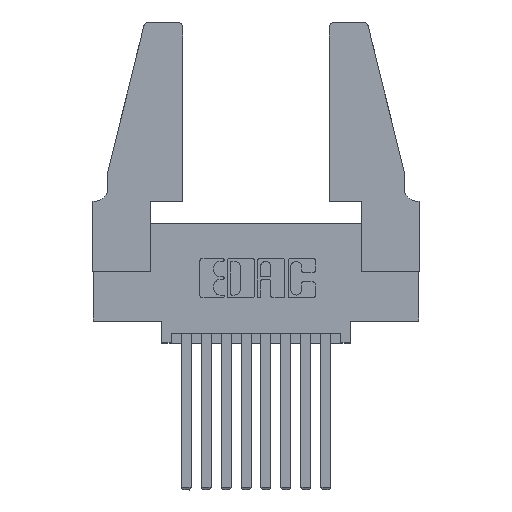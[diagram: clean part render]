
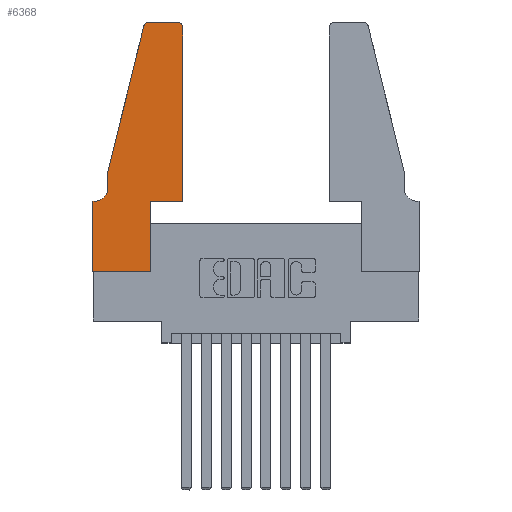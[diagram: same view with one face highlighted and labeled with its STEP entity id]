
A CAD part, top view. The second image highlights one B-rep face of the part: STEP entity #6368.
In plain terms, the highlighted planar face has unit normal (0, 0, 1).
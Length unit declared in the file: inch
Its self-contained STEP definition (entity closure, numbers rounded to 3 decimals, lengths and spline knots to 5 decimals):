
#100 = ORIENTED_EDGE ( 'NONE', *, *, #12266, .T. ) ;
#156 = VECTOR ( 'NONE', #745, 39.37008 ) ;
#252 = VERTEX_POINT ( 'NONE', #7907 ) ;
#286 = DIRECTION ( 'NONE',  ( -0.239, -0.971, 0. ) ) ;
#383 = CARTESIAN_POINT ( 'NONE',  ( 0., 0., 0.37 ) ) ;
#745 = DIRECTION ( 'NONE',  ( -1., 0., 0. ) ) ;
#772 = CARTESIAN_POINT ( 'NONE',  ( 0.0755, 0.5, 0.37 ) ) ;
#869 = CARTESIAN_POINT ( 'NONE',  ( 0.4205, 1.22, 0.37 ) ) ;
#890 = AXIS2_PLACEMENT_3D ( 'NONE', #2782, #3839, #6799 ) ;
#1001 = CARTESIAN_POINT ( 'NONE',  ( 0.284, 1.25, 0.37 ) ) ;
#1267 = CARTESIAN_POINT ( 'NONE',  ( 0.4505, 1.22, 0.37 ) ) ;
#1347 = ORIENTED_EDGE ( 'NONE', *, *, #10924, .T. ) ;
#1435 = VECTOR ( 'NONE', #3525, 39.37008 ) ;
#1840 = CARTESIAN_POINT ( 'NONE',  ( 0.4505, 0.35, 0.37 ) ) ;
#1850 = LINE ( 'NONE', #772, #5919 ) ;
#1855 = EDGE_CURVE ( 'NONE', #7371, #9687, #1850, .T. ) ;
#1903 = CARTESIAN_POINT ( 'NONE',  ( 0.0755, 0.5, 0.37 ) ) ;
#2557 = CARTESIAN_POINT ( 'NONE',  ( 0.2865, 0.35, 0.37 ) ) ;
#2782 = CARTESIAN_POINT ( 'NONE',  ( 0.0055, 0.42, 0.37 ) ) ;
#2971 = LINE ( 'NONE', #7767, #8925 ) ;
#3011 = CIRCLE ( 'NONE', #890, 0.07 ) ;
#3025 = CIRCLE ( 'NONE', #7605, 0.03 ) ;
#3317 = EDGE_CURVE ( 'NONE', #11089, #12493, #10253, .T. ) ;
#3330 = CARTESIAN_POINT ( 'NONE',  ( 0.284, 1.22, 0.37 ) ) ;
#3419 = DIRECTION ( 'NONE',  ( 1., 0., 0. ) ) ;
#3525 = DIRECTION ( 'NONE',  ( 0., -1., 0. ) ) ;
#3647 = CARTESIAN_POINT ( 'NONE',  ( 0., 0.35, 0.37 ) ) ;
#3662 = VECTOR ( 'NONE', #10313, 39.37008 ) ;
#3750 = VECTOR ( 'NONE', #286, 39.37008 ) ;
#3831 = PLANE ( 'NONE',  #8722 ) ;
#3839 = DIRECTION ( 'NONE',  ( 0., 0., -1. ) ) ;
#3955 = AXIS2_PLACEMENT_3D ( 'NONE', #3330, #9452, #3419 ) ;
#4276 = CARTESIAN_POINT ( 'NONE',  ( 0., 0.35, 0.37 ) ) ;
#4323 = VECTOR ( 'NONE', #5979, 39.37008 ) ;
#4641 = ORIENTED_EDGE ( 'NONE', *, *, #11639, .T. ) ;
#5005 = CARTESIAN_POINT ( 'NONE',  ( 0.0055, 0.35, 0.37 ) ) ;
#5473 = LINE ( 'NONE', #6293, #3750 ) ;
#5795 = DIRECTION ( 'NONE',  ( 0., 0., 1. ) ) ;
#5812 = DIRECTION ( 'NONE',  ( 1., 0., 0. ) ) ;
#5919 = VECTOR ( 'NONE', #11779, 39.37008 ) ;
#5979 = DIRECTION ( 'NONE',  ( -1., 0., 0. ) ) ;
#6196 = VECTOR ( 'NONE', #12557, 39.37008 ) ;
#6293 = CARTESIAN_POINT ( 'NONE',  ( 0.0755, 0.5, 0.37 ) ) ;
#6336 = CARTESIAN_POINT ( 'NONE',  ( 0.4505, 0.35, 0.37 ) ) ;
#6368 = ADVANCED_FACE ( 'NONE', ( #8621 ), #3831, .T. ) ;
#6444 = LINE ( 'NONE', #9816, #156 ) ;
#6614 = EDGE_CURVE ( 'NONE', #12202, #7371, #5473, .T. ) ;
#6792 = ORIENTED_EDGE ( 'NONE', *, *, #7419, .T. ) ;
#6795 = CARTESIAN_POINT ( 'NONE',  ( 0.2605, 1.25, 0.37 ) ) ;
#6799 = DIRECTION ( 'NONE',  ( -1., 0., 0. ) ) ;
#7087 = ORIENTED_EDGE ( 'NONE', *, *, #3317, .T. ) ;
#7198 = ORIENTED_EDGE ( 'NONE', *, *, #8998, .T. ) ;
#7279 = EDGE_CURVE ( 'NONE', #8082, #12202, #12154, .T. ) ;
#7371 = VERTEX_POINT ( 'NONE', #1903 ) ;
#7419 = EDGE_CURVE ( 'NONE', #9749, #12370, #2971, .T. ) ;
#7465 = ORIENTED_EDGE ( 'NONE', *, *, #1855, .T. ) ;
#7605 = AXIS2_PLACEMENT_3D ( 'NONE', #869, #12843, #5812 ) ;
#7742 = CARTESIAN_POINT ( 'NONE',  ( 0.25487, 1.22718, 0.37 ) ) ;
#7767 = CARTESIAN_POINT ( 'NONE',  ( 0., 0., 0.37 ) ) ;
#7865 = ORIENTED_EDGE ( 'NONE', *, *, #10103, .T. ) ;
#7907 = CARTESIAN_POINT ( 'NONE',  ( 0.4205, 1.25, 0.37 ) ) ;
#8082 = VERTEX_POINT ( 'NONE', #1001 ) ;
#8331 = ORIENTED_EDGE ( 'NONE', *, *, #12704, .T. ) ;
#8621 = FACE_OUTER_BOUND ( 'NONE', #10375, .T. ) ;
#8636 = CARTESIAN_POINT ( 'NONE',  ( 0.4505, 0.35, 0.37 ) ) ;
#8722 = AXIS2_PLACEMENT_3D ( 'NONE', #3647, #5795, #9675 ) ;
#8925 = VECTOR ( 'NONE', #9840, 39.37008 ) ;
#8992 = LINE ( 'NONE', #6336, #3662 ) ;
#8998 = EDGE_CURVE ( 'NONE', #12370, #10031, #10120, .T. ) ;
#9105 = CARTESIAN_POINT ( 'NONE',  ( 0.0755, 0.42, 0.37 ) ) ;
#9452 = DIRECTION ( 'NONE',  ( 0., 0., 1. ) ) ;
#9516 = CARTESIAN_POINT ( 'NONE',  ( 0., 0., 0.37 ) ) ;
#9537 = DIRECTION ( 'NONE',  ( 0., 1., 0. ) ) ;
#9675 = DIRECTION ( 'NONE',  ( 1., 0., 0. ) ) ;
#9687 = VERTEX_POINT ( 'NONE', #9105 ) ;
#9749 = VERTEX_POINT ( 'NONE', #383 ) ;
#9816 = CARTESIAN_POINT ( 'NONE',  ( 0.0755, 0.35, 0.37 ) ) ;
#9840 = DIRECTION ( 'NONE',  ( 1., 0., 0. ) ) ;
#10031 = VERTEX_POINT ( 'NONE', #10703 ) ;
#10103 = EDGE_CURVE ( 'NONE', #252, #8082, #10875, .T. ) ;
#10120 = LINE ( 'NONE', #2557, #11533 ) ;
#10202 = ORIENTED_EDGE ( 'NONE', *, *, #11139, .T. ) ;
#10253 = LINE ( 'NONE', #8636, #6196 ) ;
#10313 = DIRECTION ( 'NONE',  ( 1., 0., 0. ) ) ;
#10375 = EDGE_LOOP ( 'NONE', ( #7865, #11960, #12060, #7465, #4641, #100, #8331, #6792, #7198, #1347, #7087, #10202 ) ) ;
#10703 = CARTESIAN_POINT ( 'NONE',  ( 0.2865, 0.35, 0.37 ) ) ;
#10709 = VERTEX_POINT ( 'NONE', #5005 ) ;
#10875 = LINE ( 'NONE', #6795, #4323 ) ;
#10924 = EDGE_CURVE ( 'NONE', #10031, #11089, #8992, .T. ) ;
#11089 = VERTEX_POINT ( 'NONE', #1840 ) ;
#11139 = EDGE_CURVE ( 'NONE', #12493, #252, #3025, .T. ) ;
#11533 = VECTOR ( 'NONE', #9537, 39.37008 ) ;
#11639 = EDGE_CURVE ( 'NONE', #9687, #10709, #3011, .T. ) ;
#11779 = DIRECTION ( 'NONE',  ( 0., -1., 0. ) ) ;
#11897 = VERTEX_POINT ( 'NONE', #4276 ) ;
#11960 = ORIENTED_EDGE ( 'NONE', *, *, #7279, .T. ) ;
#12055 = CARTESIAN_POINT ( 'NONE',  ( 0.2865, 0., 0.37 ) ) ;
#12060 = ORIENTED_EDGE ( 'NONE', *, *, #6614, .T. ) ;
#12154 = CIRCLE ( 'NONE', #3955, 0.03 ) ;
#12202 = VERTEX_POINT ( 'NONE', #7742 ) ;
#12266 = EDGE_CURVE ( 'NONE', #10709, #11897, #6444, .T. ) ;
#12370 = VERTEX_POINT ( 'NONE', #12055 ) ;
#12493 = VERTEX_POINT ( 'NONE', #1267 ) ;
#12557 = DIRECTION ( 'NONE',  ( 0., 1., 0. ) ) ;
#12704 = EDGE_CURVE ( 'NONE', #11897, #9749, #12848, .T. ) ;
#12843 = DIRECTION ( 'NONE',  ( 0., 0., 1. ) ) ;
#12848 = LINE ( 'NONE', #9516, #1435 ) ;
